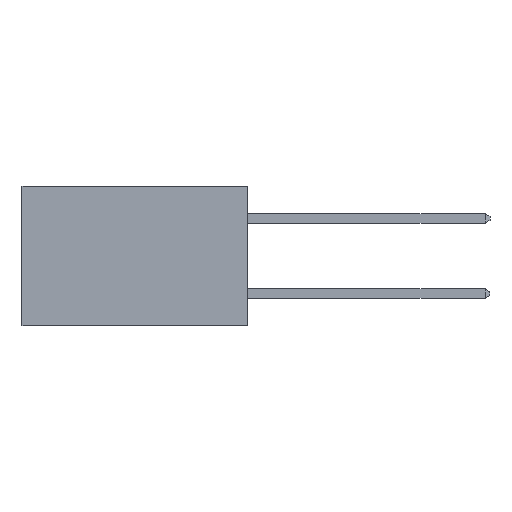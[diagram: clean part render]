
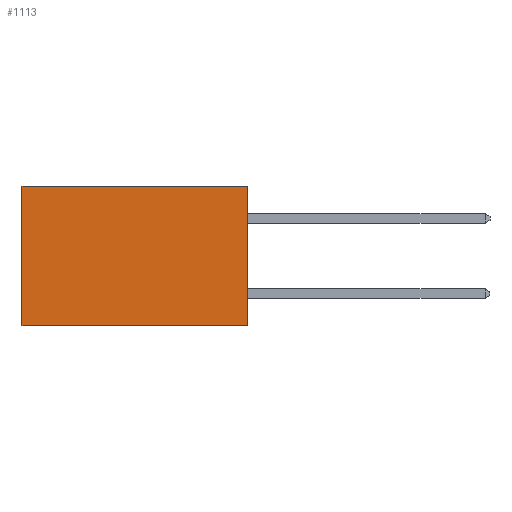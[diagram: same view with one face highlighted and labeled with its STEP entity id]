
A CAD part, left-side view. The second image highlights one B-rep face of the part: STEP entity #1113.
In plain terms, the highlighted planar face has unit normal (-1, 0, 0).
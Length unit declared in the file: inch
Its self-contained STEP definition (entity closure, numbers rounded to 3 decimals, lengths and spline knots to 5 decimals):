
#142 = DIRECTION ( 'NONE',  ( 0., 1., 0. ) ) ;
#316 = EDGE_CURVE ( 'NONE', #892, #8870, #8148, .T. ) ;
#892 = VERTEX_POINT ( 'NONE', #5699 ) ;
#1101 = EDGE_CURVE ( 'NONE', #892, #2861, #9208, .T. ) ;
#1113 = ADVANCED_FACE ( 'NONE', ( #6921 ), #5201, .F. ) ;
#1766 = ORIENTED_EDGE ( 'NONE', *, *, #1101, .T. ) ;
#2159 = ORIENTED_EDGE ( 'NONE', *, *, #5097, .T. ) ;
#2861 = VERTEX_POINT ( 'NONE', #9040 ) ;
#3089 = VECTOR ( 'NONE', #9469, 39.37008 ) ;
#3400 = CARTESIAN_POINT ( 'NONE',  ( 0.298, 0., 0. ) ) ;
#3865 = CARTESIAN_POINT ( 'NONE',  ( 0.298, 0., 0. ) ) ;
#3885 = DIRECTION ( 'NONE',  ( 0., 1., 0. ) ) ;
#4567 = DIRECTION ( 'NONE',  ( 1., 0., 0. ) ) ;
#5021 = ORIENTED_EDGE ( 'NONE', *, *, #9439, .F. ) ;
#5097 = EDGE_CURVE ( 'NONE', #2861, #5378, #5175, .T. ) ;
#5134 = DIRECTION ( 'NONE',  ( 0., 0., -1. ) ) ;
#5175 = LINE ( 'NONE', #8400, #6573 ) ;
#5201 = PLANE ( 'NONE',  #5407 ) ;
#5378 = VERTEX_POINT ( 'NONE', #6756 ) ;
#5407 = AXIS2_PLACEMENT_3D ( 'NONE', #3400, #4567, #5134 ) ;
#5699 = CARTESIAN_POINT ( 'NONE',  ( 0.298, 0., 0. ) ) ;
#6573 = VECTOR ( 'NONE', #12230, 39.37008 ) ;
#6607 = VECTOR ( 'NONE', #3885, 39.37008 ) ;
#6756 = CARTESIAN_POINT ( 'NONE',  ( 0.298, 0.6, -0.37 ) ) ;
#6921 = FACE_OUTER_BOUND ( 'NONE', #11818, .T. ) ;
#7126 = ORIENTED_EDGE ( 'NONE', *, *, #316, .F. ) ;
#7946 = CARTESIAN_POINT ( 'NONE',  ( 0.298, 0., -0.37 ) ) ;
#8148 = LINE ( 'NONE', #9850, #3089 ) ;
#8349 = CARTESIAN_POINT ( 'NONE',  ( 0.298, 0., -0.37 ) ) ;
#8400 = CARTESIAN_POINT ( 'NONE',  ( 0.298, 0.6, 0. ) ) ;
#8870 = VERTEX_POINT ( 'NONE', #8349 ) ;
#9040 = CARTESIAN_POINT ( 'NONE',  ( 0.298, 0.6, 0. ) ) ;
#9208 = LINE ( 'NONE', #3865, #6607 ) ;
#9439 = EDGE_CURVE ( 'NONE', #8870, #5378, #12243, .T. ) ;
#9469 = DIRECTION ( 'NONE',  ( 0., 0., -1. ) ) ;
#9850 = CARTESIAN_POINT ( 'NONE',  ( 0.298, 0., 0. ) ) ;
#9930 = VECTOR ( 'NONE', #142, 39.37008 ) ;
#11818 = EDGE_LOOP ( 'NONE', ( #2159, #5021, #7126, #1766 ) ) ;
#12230 = DIRECTION ( 'NONE',  ( 0., 0., -1. ) ) ;
#12243 = LINE ( 'NONE', #7946, #9930 ) ;
